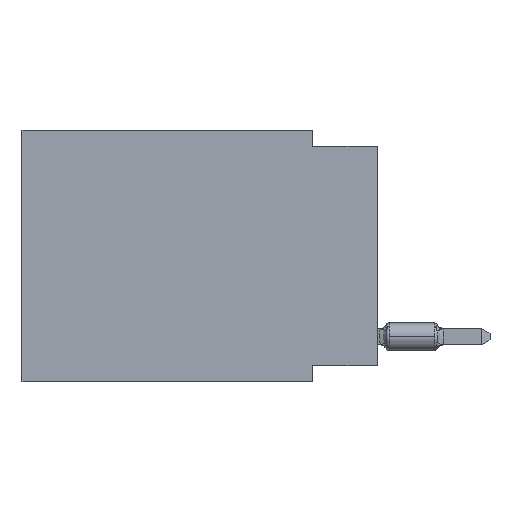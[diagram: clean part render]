
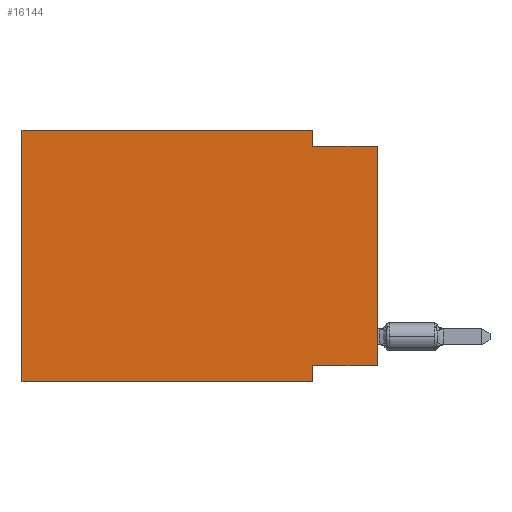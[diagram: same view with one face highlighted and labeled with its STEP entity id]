
A CAD part, left-side view. The second image highlights one B-rep face of the part: STEP entity #16144.
In plain terms, the highlighted planar face has unit normal (-1, 0, 0).
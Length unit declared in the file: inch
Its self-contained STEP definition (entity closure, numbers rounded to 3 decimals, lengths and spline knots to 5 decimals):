
#302 = VERTEX_POINT ( 'NONE', #15436 ) ;
#1220 = DIRECTION ( 'NONE',  ( 0., -1., 0. ) ) ;
#1231 = LINE ( 'NONE', #6893, #6549 ) ;
#1333 = EDGE_CURVE ( 'NONE', #6832, #1766, #7691, .T. ) ;
#1455 = CARTESIAN_POINT ( 'NONE',  ( 0., 0.55, 0. ) ) ;
#1494 = EDGE_CURVE ( 'NONE', #4873, #6832, #2847, .T. ) ;
#1643 = ORIENTED_EDGE ( 'NONE', *, *, #16066, .F. ) ;
#1766 = VERTEX_POINT ( 'NONE', #16073 ) ;
#2847 = LINE ( 'NONE', #1455, #16784 ) ;
#3022 = CARTESIAN_POINT ( 'NONE',  ( 0., 0., 0. ) ) ;
#3073 = FACE_OUTER_BOUND ( 'NONE', #16565, .T. ) ;
#3227 = ORIENTED_EDGE ( 'NONE', *, *, #1333, .F. ) ;
#3360 = EDGE_CURVE ( 'NONE', #5138, #302, #15533, .T. ) ;
#3847 = VECTOR ( 'NONE', #8640, 39.37008 ) ;
#4255 = ORIENTED_EDGE ( 'NONE', *, *, #4511, .F. ) ;
#4460 = DIRECTION ( 'NONE',  ( 1., 0., 0. ) ) ;
#4511 = EDGE_CURVE ( 'NONE', #1766, #15995, #12854, .T. ) ;
#4873 = VERTEX_POINT ( 'NONE', #8492 ) ;
#5083 = EDGE_CURVE ( 'NONE', #5138, #10591, #8950, .T. ) ;
#5138 = VERTEX_POINT ( 'NONE', #8035 ) ;
#5548 = DIRECTION ( 'NONE',  ( 0., 1., 0. ) ) ;
#5568 = LINE ( 'NONE', #8444, #10343 ) ;
#6023 = CARTESIAN_POINT ( 'NONE',  ( 0., 0.55, 0. ) ) ;
#6110 = CARTESIAN_POINT ( 'NONE',  ( 0., 0.55, 0. ) ) ;
#6549 = VECTOR ( 'NONE', #10975, 39.37008 ) ;
#6832 = VERTEX_POINT ( 'NONE', #6110 ) ;
#6864 = DIRECTION ( 'NONE',  ( 0., 0., -1. ) ) ;
#6893 = CARTESIAN_POINT ( 'NONE',  ( 0., 0.1, -0.39 ) ) ;
#7438 = VECTOR ( 'NONE', #14589, 39.37008 ) ;
#7691 = LINE ( 'NONE', #6023, #9098 ) ;
#8035 = CARTESIAN_POINT ( 'NONE',  ( 0., 0., -0.365 ) ) ;
#8444 = CARTESIAN_POINT ( 'NONE',  ( 0., 0., -0.025 ) ) ;
#8492 = CARTESIAN_POINT ( 'NONE',  ( 0., 0.55, -0.39 ) ) ;
#8640 = DIRECTION ( 'NONE',  ( 0., -1., 0. ) ) ;
#8820 = CARTESIAN_POINT ( 'NONE',  ( 0., 0., -0.025 ) ) ;
#8909 = CARTESIAN_POINT ( 'NONE',  ( 0., 0.55, 0. ) ) ;
#8950 = LINE ( 'NONE', #3022, #7438 ) ;
#9098 = VECTOR ( 'NONE', #14907, 39.37008 ) ;
#9824 = ORIENTED_EDGE ( 'NONE', *, *, #15007, .T. ) ;
#9853 = ORIENTED_EDGE ( 'NONE', *, *, #10847, .F. ) ;
#10119 = DIRECTION ( 'NONE',  ( 0., 0., -1. ) ) ;
#10343 = VECTOR ( 'NONE', #1220, 39.37008 ) ;
#10591 = VERTEX_POINT ( 'NONE', #8820 ) ;
#10847 = EDGE_CURVE ( 'NONE', #15995, #10591, #5568, .T. ) ;
#10975 = DIRECTION ( 'NONE',  ( 0., 0., -1. ) ) ;
#11504 = PLANE ( 'NONE',  #18039 ) ;
#11799 = ORIENTED_EDGE ( 'NONE', *, *, #1494, .F. ) ;
#11863 = VECTOR ( 'NONE', #6864, 39.37008 ) ;
#11930 = ORIENTED_EDGE ( 'NONE', *, *, #3360, .F. ) ;
#12411 = CARTESIAN_POINT ( 'NONE',  ( 0., 0., -0.365 ) ) ;
#12854 = LINE ( 'NONE', #14064, #11863 ) ;
#13805 = ORIENTED_EDGE ( 'NONE', *, *, #5083, .T. ) ;
#14055 = DIRECTION ( 'NONE',  ( 0., 0., 1. ) ) ;
#14064 = CARTESIAN_POINT ( 'NONE',  ( 0., 0.1, 0. ) ) ;
#14589 = DIRECTION ( 'NONE',  ( 0., 0., 1. ) ) ;
#14907 = DIRECTION ( 'NONE',  ( 0., -1., 0. ) ) ;
#15007 = EDGE_CURVE ( 'NONE', #4873, #15909, #15652, .T. ) ;
#15436 = CARTESIAN_POINT ( 'NONE',  ( 0., 0.1, -0.365 ) ) ;
#15533 = LINE ( 'NONE', #12411, #15710 ) ;
#15652 = LINE ( 'NONE', #17029, #3847 ) ;
#15710 = VECTOR ( 'NONE', #5548, 39.37008 ) ;
#15909 = VERTEX_POINT ( 'NONE', #16413 ) ;
#15995 = VERTEX_POINT ( 'NONE', #16685 ) ;
#16066 = EDGE_CURVE ( 'NONE', #302, #15909, #1231, .T. ) ;
#16073 = CARTESIAN_POINT ( 'NONE',  ( 0., 0.1, 0. ) ) ;
#16144 = ADVANCED_FACE ( 'NONE', ( #3073 ), #11504, .F. ) ;
#16413 = CARTESIAN_POINT ( 'NONE',  ( 0., 0.1, -0.39 ) ) ;
#16565 = EDGE_LOOP ( 'NONE', ( #13805, #9853, #4255, #3227, #11799, #9824, #1643, #11930 ) ) ;
#16685 = CARTESIAN_POINT ( 'NONE',  ( 0., 0.1, -0.025 ) ) ;
#16784 = VECTOR ( 'NONE', #14055, 39.37008 ) ;
#17029 = CARTESIAN_POINT ( 'NONE',  ( 0., 0.55, -0.39 ) ) ;
#18039 = AXIS2_PLACEMENT_3D ( 'NONE', #8909, #4460, #10119 ) ;
